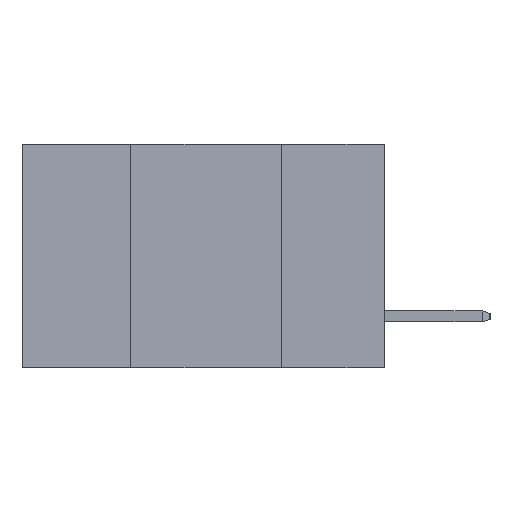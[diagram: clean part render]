
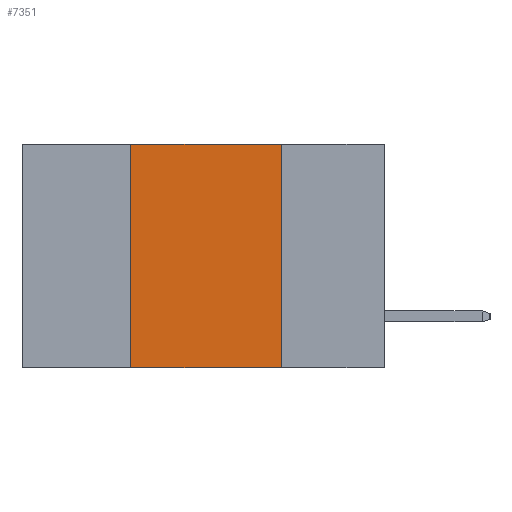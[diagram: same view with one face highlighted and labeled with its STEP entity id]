
A CAD part, left-side view. The second image highlights one B-rep face of the part: STEP entity #7351.
In plain terms, the highlighted planar face has unit normal (-1, 0, 0).
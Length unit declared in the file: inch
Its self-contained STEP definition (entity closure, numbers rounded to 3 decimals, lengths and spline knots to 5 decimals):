
#159 = EDGE_CURVE ( 'NONE', #5916, #5834, #22268, .T. ) ;
#635 = DIRECTION ( 'NONE',  ( 0., -1., 0. ) ) ;
#1293 = ORIENTED_EDGE ( 'NONE', *, *, #2934, .F. ) ;
#1462 = CARTESIAN_POINT ( 'NONE',  ( 0., 0.42, 0. ) ) ;
#1577 = ORIENTED_EDGE ( 'NONE', *, *, #15811, .T. ) ;
#2796 = CARTESIAN_POINT ( 'NONE',  ( 0., 0.6, 0. ) ) ;
#2934 = EDGE_CURVE ( 'NONE', #5834, #19829, #9758, .T. ) ;
#3692 = CARTESIAN_POINT ( 'NONE',  ( 0., 0.17, 0. ) ) ;
#3988 = ORIENTED_EDGE ( 'NONE', *, *, #15381, .F. ) ;
#5035 = VECTOR ( 'NONE', #13302, 39.37008 ) ;
#5834 = VERTEX_POINT ( 'NONE', #3692 ) ;
#5916 = VERTEX_POINT ( 'NONE', #1462 ) ;
#6503 = CARTESIAN_POINT ( 'NONE',  ( 0., 0.17, -0.37 ) ) ;
#7351 = ADVANCED_FACE ( 'NONE', ( #12594 ), #13981, .F. ) ;
#8544 = VECTOR ( 'NONE', #635, 39.37008 ) ;
#8558 = CARTESIAN_POINT ( 'NONE',  ( 0., 0.42, -0.37 ) ) ;
#9758 = LINE ( 'NONE', #13709, #5035 ) ;
#10358 = DIRECTION ( 'NONE',  ( 0., 0., 1. ) ) ;
#12404 = VECTOR ( 'NONE', #17717, 39.37008 ) ;
#12594 = FACE_OUTER_BOUND ( 'NONE', #13887, .T. ) ;
#13019 = AXIS2_PLACEMENT_3D ( 'NONE', #14272, #15290, #14968 ) ;
#13254 = CARTESIAN_POINT ( 'NONE',  ( 0., 0.6, -0.37 ) ) ;
#13302 = DIRECTION ( 'NONE',  ( 0., 0., -1. ) ) ;
#13709 = CARTESIAN_POINT ( 'NONE',  ( 0., 0.17, -0.37 ) ) ;
#13887 = EDGE_LOOP ( 'NONE', ( #1293, #18458, #3988, #1577 ) ) ;
#13981 = PLANE ( 'NONE',  #13019 ) ;
#14078 = CARTESIAN_POINT ( 'NONE',  ( 0., 0.42, -0.37 ) ) ;
#14272 = CARTESIAN_POINT ( 'NONE',  ( 0., 0.6, 0. ) ) ;
#14968 = DIRECTION ( 'NONE',  ( 0., 0., -1. ) ) ;
#15290 = DIRECTION ( 'NONE',  ( 1., 0., 0. ) ) ;
#15381 = EDGE_CURVE ( 'NONE', #20695, #5916, #16249, .T. ) ;
#15811 = EDGE_CURVE ( 'NONE', #20695, #19829, #22043, .T. ) ;
#16249 = LINE ( 'NONE', #8558, #20119 ) ;
#17717 = DIRECTION ( 'NONE',  ( 0., -1., 0. ) ) ;
#18458 = ORIENTED_EDGE ( 'NONE', *, *, #159, .F. ) ;
#19829 = VERTEX_POINT ( 'NONE', #6503 ) ;
#20119 = VECTOR ( 'NONE', #10358, 39.37008 ) ;
#20695 = VERTEX_POINT ( 'NONE', #14078 ) ;
#22043 = LINE ( 'NONE', #13254, #8544 ) ;
#22268 = LINE ( 'NONE', #2796, #12404 ) ;
